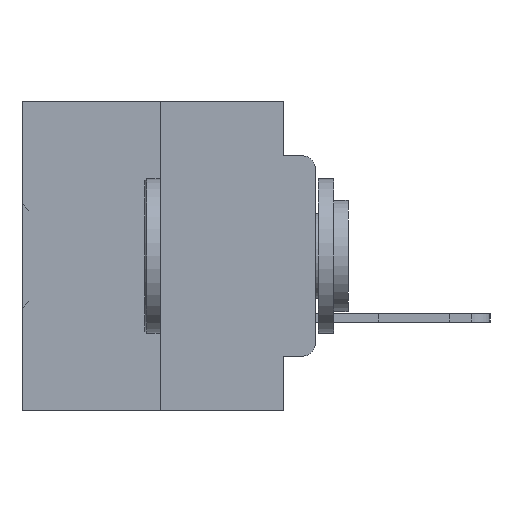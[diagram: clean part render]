
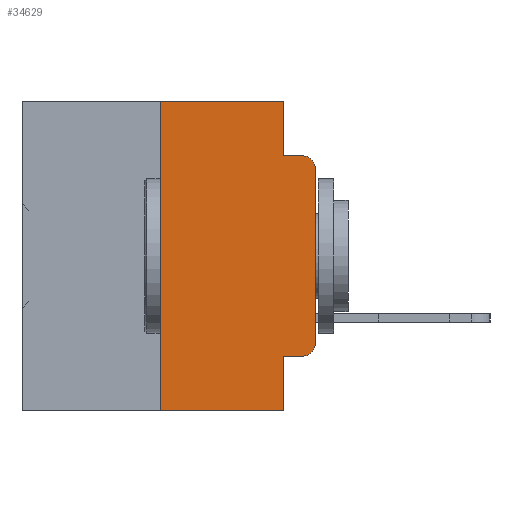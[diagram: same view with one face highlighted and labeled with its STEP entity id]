
A CAD part, left-side view. The second image highlights one B-rep face of the part: STEP entity #34629.
In plain terms, the highlighted planar face has unit normal (-1, 0, 0).
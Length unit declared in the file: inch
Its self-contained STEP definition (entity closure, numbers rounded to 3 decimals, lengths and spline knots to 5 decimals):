
#260 = LINE ( 'NONE', #22692, #29334 ) ;
#1274 = ORIENTED_EDGE ( 'NONE', *, *, #19074, .F. ) ;
#2454 = CARTESIAN_POINT ( 'NONE',  ( 0., 0.02, -0.3915 ) ) ;
#2741 = EDGE_CURVE ( 'NONE', #24371, #23050, #3208, .T. ) ;
#3151 = VERTEX_POINT ( 'NONE', #14296 ) ;
#3208 = LINE ( 'NONE', #8138, #32231 ) ;
#4924 = VERTEX_POINT ( 'NONE', #8326 ) ;
#5354 = DIRECTION ( 'NONE',  ( 0., 0., -1. ) ) ;
#5649 = CARTESIAN_POINT ( 'NONE',  ( 0., 0.02, -0.1085 ) ) ;
#6221 = CARTESIAN_POINT ( 'NONE',  ( 0., 0.051, -0.5 ) ) ;
#7328 = EDGE_CURVE ( 'NONE', #30196, #24371, #31331, .T. ) ;
#7372 = CIRCLE ( 'NONE', #23266, 0.02 ) ;
#7828 = ORIENTED_EDGE ( 'NONE', *, *, #26362, .F. ) ;
#8138 = CARTESIAN_POINT ( 'NONE',  ( 0., 0., 0. ) ) ;
#8249 = DIRECTION ( 'NONE',  ( 0., 0., 1. ) ) ;
#8323 = CARTESIAN_POINT ( 'NONE',  ( 0., 0., -0.3915 ) ) ;
#8326 = CARTESIAN_POINT ( 'NONE',  ( 0., 0.02, -0.0885 ) ) ;
#8567 = DIRECTION ( 'NONE',  ( 0., 0., -1. ) ) ;
#9928 = LINE ( 'NONE', #30924, #32135 ) ;
#10023 = VECTOR ( 'NONE', #19042, 39.37008 ) ;
#10207 = DIRECTION ( 'NONE',  ( 0., 0., 1. ) ) ;
#10415 = LINE ( 'NONE', #14106, #24969 ) ;
#10914 = LINE ( 'NONE', #13038, #10023 ) ;
#10952 = VECTOR ( 'NONE', #11136, 39.37008 ) ;
#11136 = DIRECTION ( 'NONE',  ( 0., -1., 0. ) ) ;
#11142 = CARTESIAN_POINT ( 'NONE',  ( 0., 0.051, -0.0885 ) ) ;
#11280 = VERTEX_POINT ( 'NONE', #36260 ) ;
#12616 = ORIENTED_EDGE ( 'NONE', *, *, #28721, .F. ) ;
#12813 = CARTESIAN_POINT ( 'NONE',  ( 0., 0.473, 0. ) ) ;
#13038 = CARTESIAN_POINT ( 'NONE',  ( 0., 0.051, 0. ) ) ;
#13839 = FACE_OUTER_BOUND ( 'NONE', #27614, .T. ) ;
#14082 = CARTESIAN_POINT ( 'NONE',  ( 0., 0.473, 0. ) ) ;
#14106 = CARTESIAN_POINT ( 'NONE',  ( 0., 0.473, -0.5 ) ) ;
#14296 = CARTESIAN_POINT ( 'NONE',  ( 0., 0.051, -0.4115 ) ) ;
#14510 = ORIENTED_EDGE ( 'NONE', *, *, #22921, .F. ) ;
#14927 = EDGE_CURVE ( 'NONE', #25861, #21547, #10415, .T. ) ;
#15616 = PLANE ( 'NONE',  #29409 ) ;
#15752 = DIRECTION ( 'NONE',  ( 0., 0., -1. ) ) ;
#16633 = ORIENTED_EDGE ( 'NONE', *, *, #17121, .T. ) ;
#17058 = DIRECTION ( 'NONE',  ( 0., -1., 0. ) ) ;
#17121 = EDGE_CURVE ( 'NONE', #3151, #30196, #33671, .T. ) ;
#17460 = CARTESIAN_POINT ( 'NONE',  ( 0., 0.25, -0.5 ) ) ;
#18735 = LINE ( 'NONE', #14082, #10952 ) ;
#19042 = DIRECTION ( 'NONE',  ( 0., 0., -1. ) ) ;
#19074 = EDGE_CURVE ( 'NONE', #3151, #21547, #9928, .T. ) ;
#19407 = ORIENTED_EDGE ( 'NONE', *, *, #7328, .T. ) ;
#19856 = ORIENTED_EDGE ( 'NONE', *, *, #2741, .T. ) ;
#20956 = DIRECTION ( 'NONE',  ( 0., -1., 0. ) ) ;
#21547 = VERTEX_POINT ( 'NONE', #6221 ) ;
#21771 = CARTESIAN_POINT ( 'NONE',  ( 0., 0.25, 0. ) ) ;
#22160 = VECTOR ( 'NONE', #10207, 39.37008 ) ;
#22692 = CARTESIAN_POINT ( 'NONE',  ( 0., 0.051, -0.0885 ) ) ;
#22765 = DIRECTION ( 'NONE',  ( -1., 0., 0. ) ) ;
#22885 = ORIENTED_EDGE ( 'NONE', *, *, #26809, .F. ) ;
#22921 = EDGE_CURVE ( 'NONE', #25861, #32378, #30721, .T. ) ;
#23050 = VERTEX_POINT ( 'NONE', #33897 ) ;
#23266 = AXIS2_PLACEMENT_3D ( 'NONE', #5649, #25955, #8567 ) ;
#24371 = VERTEX_POINT ( 'NONE', #8323 ) ;
#24969 = VECTOR ( 'NONE', #17058, 39.37008 ) ;
#25861 = VERTEX_POINT ( 'NONE', #17460 ) ;
#25955 = DIRECTION ( 'NONE',  ( -1., 0., 0. ) ) ;
#25984 = VECTOR ( 'NONE', #20956, 39.37008 ) ;
#26362 = EDGE_CURVE ( 'NONE', #32378, #11280, #18735, .T. ) ;
#26809 = EDGE_CURVE ( 'NONE', #11280, #29937, #10914, .T. ) ;
#27614 = EDGE_LOOP ( 'NONE', ( #19856, #28329, #12616, #22885, #7828, #14510, #36985, #1274, #16633, #19407 ) ) ;
#28234 = AXIS2_PLACEMENT_3D ( 'NONE', #2454, #22765, #5354 ) ;
#28329 = ORIENTED_EDGE ( 'NONE', *, *, #30641, .T. ) ;
#28721 = EDGE_CURVE ( 'NONE', #29937, #4924, #260, .T. ) ;
#29334 = VECTOR ( 'NONE', #34308, 39.37008 ) ;
#29409 = AXIS2_PLACEMENT_3D ( 'NONE', #12813, #33073, #15752 ) ;
#29937 = VERTEX_POINT ( 'NONE', #11142 ) ;
#30196 = VERTEX_POINT ( 'NONE', #35344 ) ;
#30641 = EDGE_CURVE ( 'NONE', #23050, #4924, #7372, .T. ) ;
#30721 = LINE ( 'NONE', #21771, #22160 ) ;
#30924 = CARTESIAN_POINT ( 'NONE',  ( 0., 0.051, 0. ) ) ;
#31331 = CIRCLE ( 'NONE', #28234, 0.02 ) ;
#31920 = CARTESIAN_POINT ( 'NONE',  ( 0., 0.25, 0. ) ) ;
#32135 = VECTOR ( 'NONE', #33861, 39.37008 ) ;
#32231 = VECTOR ( 'NONE', #8249, 39.37008 ) ;
#32378 = VERTEX_POINT ( 'NONE', #31920 ) ;
#32438 = CARTESIAN_POINT ( 'NONE',  ( 0., 0.051, -0.4115 ) ) ;
#33073 = DIRECTION ( 'NONE',  ( 1., 0., 0. ) ) ;
#33671 = LINE ( 'NONE', #32438, #25984 ) ;
#33861 = DIRECTION ( 'NONE',  ( 0., 0., -1. ) ) ;
#33897 = CARTESIAN_POINT ( 'NONE',  ( 0., 0., -0.1085 ) ) ;
#34308 = DIRECTION ( 'NONE',  ( 0., -1., 0. ) ) ;
#34629 = ADVANCED_FACE ( 'NONE', ( #13839 ), #15616, .F. ) ;
#35344 = CARTESIAN_POINT ( 'NONE',  ( 0., 0.02, -0.4115 ) ) ;
#36260 = CARTESIAN_POINT ( 'NONE',  ( 0., 0.051, 0. ) ) ;
#36985 = ORIENTED_EDGE ( 'NONE', *, *, #14927, .T. ) ;
